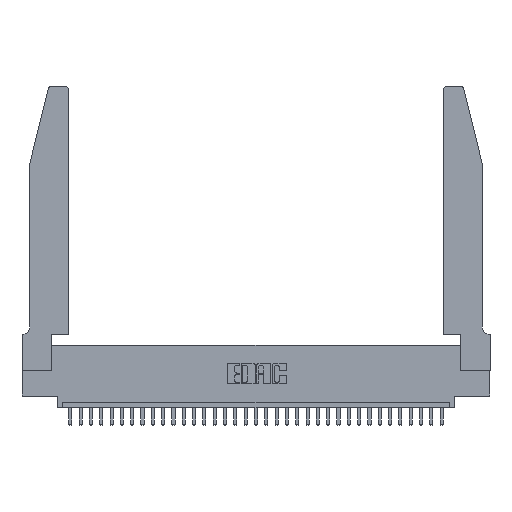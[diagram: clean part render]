
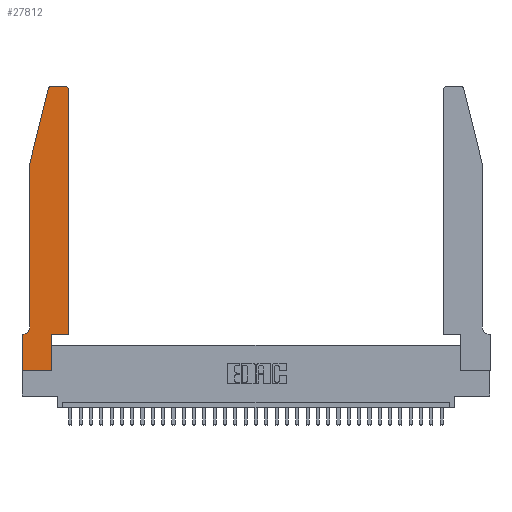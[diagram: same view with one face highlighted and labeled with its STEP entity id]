
A CAD part, top view. The second image highlights one B-rep face of the part: STEP entity #27812.
In plain terms, the highlighted planar face has unit normal (0, 0, 1).
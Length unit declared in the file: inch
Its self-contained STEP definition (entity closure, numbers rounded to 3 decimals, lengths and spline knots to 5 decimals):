
#266 = ORIENTED_EDGE ( 'NONE', *, *, #30180, .T. ) ;
#392 = CARTESIAN_POINT ( 'NONE',  ( 0., 0., 0.37 ) ) ;
#1589 = AXIS2_PLACEMENT_3D ( 'NONE', #27296, #19616, #20511 ) ;
#1729 = DIRECTION ( 'NONE',  ( 1., 0., 0. ) ) ;
#2429 = CARTESIAN_POINT ( 'NONE',  ( 0.4505, 0.35, 0.37 ) ) ;
#2667 = VECTOR ( 'NONE', #18478, 39.37008 ) ;
#3208 = DIRECTION ( 'NONE',  ( 1., 0., 0. ) ) ;
#3581 = AXIS2_PLACEMENT_3D ( 'NONE', #25454, #25216, #28143 ) ;
#3733 = ORIENTED_EDGE ( 'NONE', *, *, #22872, .T. ) ;
#3806 = LINE ( 'NONE', #31185, #23661 ) ;
#4222 = VERTEX_POINT ( 'NONE', #8807 ) ;
#4821 = ORIENTED_EDGE ( 'NONE', *, *, #30232, .T. ) ;
#5045 = DIRECTION ( 'NONE',  ( -1., 0., 0. ) ) ;
#5178 = CARTESIAN_POINT ( 'NONE',  ( 0.2865, 0.35, 0.37 ) ) ;
#5508 = DIRECTION ( 'NONE',  ( 1., 0., 0. ) ) ;
#5758 = AXIS2_PLACEMENT_3D ( 'NONE', #14171, #6348, #1729 ) ;
#5849 = EDGE_CURVE ( 'NONE', #7033, #22258, #25144, .T. ) ;
#6348 = DIRECTION ( 'NONE',  ( 0., 0., 1. ) ) ;
#6716 = EDGE_LOOP ( 'NONE', ( #25129, #266, #18351, #30463, #3733, #25758, #4821, #21590, #21568, #26808, #32582, #30719 ) ) ;
#6717 = CIRCLE ( 'NONE', #5758, 0.03 ) ;
#7033 = VERTEX_POINT ( 'NONE', #31130 ) ;
#7075 = DIRECTION ( 'NONE',  ( 0., -1., 0. ) ) ;
#7706 = VECTOR ( 'NONE', #7075, 39.37008 ) ;
#8110 = LINE ( 'NONE', #392, #13006 ) ;
#8215 = VERTEX_POINT ( 'NONE', #5178 ) ;
#8658 = CARTESIAN_POINT ( 'NONE',  ( 0.4505, 0.35, 0.37 ) ) ;
#8755 = DIRECTION ( 'NONE',  ( 0., 1., 0. ) ) ;
#8807 = CARTESIAN_POINT ( 'NONE',  ( 0.0055, 0.35, 0.37 ) ) ;
#9019 = CARTESIAN_POINT ( 'NONE',  ( 0.0755, 0.42, 0.37 ) ) ;
#9704 = CARTESIAN_POINT ( 'NONE',  ( 0., 0., 0.37 ) ) ;
#10509 = CARTESIAN_POINT ( 'NONE',  ( 0.2865, 0., 0.37 ) ) ;
#10647 = CARTESIAN_POINT ( 'NONE',  ( 0., 0.35, 0.37 ) ) ;
#10884 = CARTESIAN_POINT ( 'NONE',  ( 0.0755, 0.35, 0.37 ) ) ;
#11744 = LINE ( 'NONE', #17496, #7706 ) ;
#11885 = VECTOR ( 'NONE', #8755, 39.37008 ) ;
#12078 = EDGE_CURVE ( 'NONE', #8215, #31180, #20631, .T. ) ;
#12309 = LINE ( 'NONE', #24266, #11885 ) ;
#13006 = VECTOR ( 'NONE', #18876, 39.37008 ) ;
#14171 = CARTESIAN_POINT ( 'NONE',  ( 0.4205, 2.72, 0.37 ) ) ;
#15420 = EDGE_CURVE ( 'NONE', #24755, #8215, #12309, .T. ) ;
#15890 = DIRECTION ( 'NONE',  ( -0.239, -0.971, 0. ) ) ;
#16211 = EDGE_CURVE ( 'NONE', #31180, #19645, #29278, .T. ) ;
#16220 = CARTESIAN_POINT ( 'NONE',  ( 0., 0., 0.37 ) ) ;
#16305 = CARTESIAN_POINT ( 'NONE',  ( 0.4505, 2.72, 0.37 ) ) ;
#16344 = DIRECTION ( 'NONE',  ( 0., 1., 0. ) ) ;
#16810 = VERTEX_POINT ( 'NONE', #9019 ) ;
#17269 = LINE ( 'NONE', #10884, #2667 ) ;
#17496 = CARTESIAN_POINT ( 'NONE',  ( 0.0755, 2., 0.37 ) ) ;
#18108 = DIRECTION ( 'NONE',  ( 0., 0., 1. ) ) ;
#18301 = VERTEX_POINT ( 'NONE', #31705 ) ;
#18351 = ORIENTED_EDGE ( 'NONE', *, *, #27890, .T. ) ;
#18459 = CARTESIAN_POINT ( 'NONE',  ( 0.2605, 2.75, 0.37 ) ) ;
#18478 = DIRECTION ( 'NONE',  ( -1., 0., 0. ) ) ;
#18748 = VERTEX_POINT ( 'NONE', #24058 ) ;
#18788 = VECTOR ( 'NONE', #32887, 39.37008 ) ;
#18876 = DIRECTION ( 'NONE',  ( 0., -1., 0. ) ) ;
#19616 = DIRECTION ( 'NONE',  ( 0., 0., -1. ) ) ;
#19645 = VERTEX_POINT ( 'NONE', #16305 ) ;
#20011 = PLANE ( 'NONE',  #3581 ) ;
#20511 = DIRECTION ( 'NONE',  ( -1., 0., 0. ) ) ;
#20631 = LINE ( 'NONE', #8658, #32358 ) ;
#21262 = AXIS2_PLACEMENT_3D ( 'NONE', #26028, #18108, #5508 ) ;
#21568 = ORIENTED_EDGE ( 'NONE', *, *, #15420, .T. ) ;
#21590 = ORIENTED_EDGE ( 'NONE', *, *, #32017, .T. ) ;
#22012 = VECTOR ( 'NONE', #16344, 39.37008 ) ;
#22258 = VERTEX_POINT ( 'NONE', #27885 ) ;
#22872 = EDGE_CURVE ( 'NONE', #16810, #4222, #31207, .T. ) ;
#22965 = CIRCLE ( 'NONE', #21262, 0.03 ) ;
#23661 = VECTOR ( 'NONE', #15890, 39.37008 ) ;
#23811 = VERTEX_POINT ( 'NONE', #10647 ) ;
#24058 = CARTESIAN_POINT ( 'NONE',  ( 0.0755, 2., 0.37 ) ) ;
#24266 = CARTESIAN_POINT ( 'NONE',  ( 0.2865, 0.35, 0.37 ) ) ;
#24613 = EDGE_CURVE ( 'NONE', #18748, #16810, #11744, .T. ) ;
#24742 = VECTOR ( 'NONE', #5045, 39.37008 ) ;
#24755 = VERTEX_POINT ( 'NONE', #10509 ) ;
#25129 = ORIENTED_EDGE ( 'NONE', *, *, #5849, .T. ) ;
#25144 = LINE ( 'NONE', #18459, #24742 ) ;
#25216 = DIRECTION ( 'NONE',  ( 0., 0., 1. ) ) ;
#25454 = CARTESIAN_POINT ( 'NONE',  ( 0., 0.35, 0.37 ) ) ;
#25758 = ORIENTED_EDGE ( 'NONE', *, *, #26678, .T. ) ;
#26028 = CARTESIAN_POINT ( 'NONE',  ( 0.284, 2.72, 0.37 ) ) ;
#26504 = LINE ( 'NONE', #9704, #18788 ) ;
#26678 = EDGE_CURVE ( 'NONE', #4222, #23811, #17269, .T. ) ;
#26808 = ORIENTED_EDGE ( 'NONE', *, *, #12078, .T. ) ;
#26931 = EDGE_CURVE ( 'NONE', #19645, #7033, #6717, .T. ) ;
#27296 = CARTESIAN_POINT ( 'NONE',  ( 0.0055, 0.42, 0.37 ) ) ;
#27812 = ADVANCED_FACE ( 'NONE', ( #33395 ), #20011, .T. ) ;
#27885 = CARTESIAN_POINT ( 'NONE',  ( 0.284, 2.75, 0.37 ) ) ;
#27890 = EDGE_CURVE ( 'NONE', #18301, #18748, #3806, .T. ) ;
#28143 = DIRECTION ( 'NONE',  ( 1., 0., 0. ) ) ;
#29278 = LINE ( 'NONE', #29767, #22012 ) ;
#29767 = CARTESIAN_POINT ( 'NONE',  ( 0.4505, 0.35, 0.37 ) ) ;
#30180 = EDGE_CURVE ( 'NONE', #22258, #18301, #22965, .T. ) ;
#30232 = EDGE_CURVE ( 'NONE', #23811, #32316, #8110, .T. ) ;
#30463 = ORIENTED_EDGE ( 'NONE', *, *, #24613, .T. ) ;
#30719 = ORIENTED_EDGE ( 'NONE', *, *, #26931, .T. ) ;
#31130 = CARTESIAN_POINT ( 'NONE',  ( 0.4205, 2.75, 0.37 ) ) ;
#31180 = VERTEX_POINT ( 'NONE', #2429 ) ;
#31185 = CARTESIAN_POINT ( 'NONE',  ( 0.0755, 2., 0.37 ) ) ;
#31207 = CIRCLE ( 'NONE', #1589, 0.07 ) ;
#31705 = CARTESIAN_POINT ( 'NONE',  ( 0.25487, 2.72718, 0.37 ) ) ;
#32017 = EDGE_CURVE ( 'NONE', #32316, #24755, #26504, .T. ) ;
#32316 = VERTEX_POINT ( 'NONE', #16220 ) ;
#32358 = VECTOR ( 'NONE', #3208, 39.37008 ) ;
#32582 = ORIENTED_EDGE ( 'NONE', *, *, #16211, .T. ) ;
#32887 = DIRECTION ( 'NONE',  ( 1., 0., 0. ) ) ;
#33395 = FACE_OUTER_BOUND ( 'NONE', #6716, .T. ) ;
